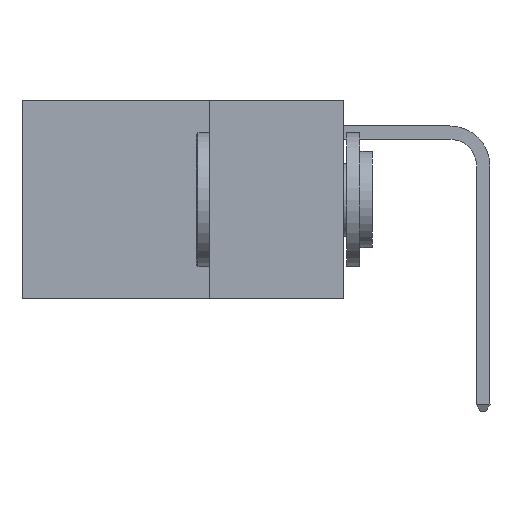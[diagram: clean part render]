
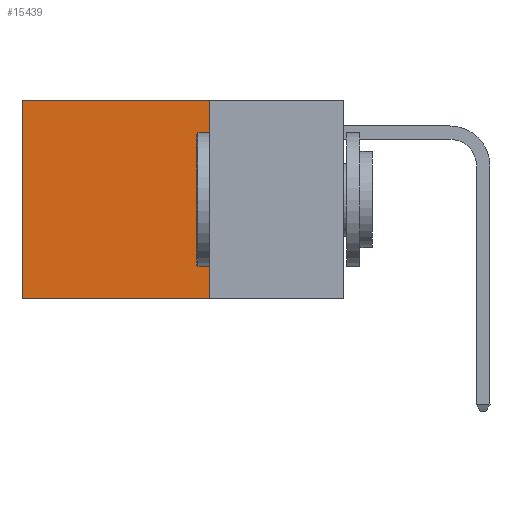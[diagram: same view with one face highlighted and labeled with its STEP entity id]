
A CAD part, left-side view. The second image highlights one B-rep face of the part: STEP entity #15439.
In plain terms, the highlighted planar face has unit normal (-1, 0, 0).
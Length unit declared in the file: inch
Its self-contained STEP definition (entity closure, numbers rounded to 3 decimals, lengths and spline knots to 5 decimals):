
#199 = LINE ( 'NONE', #15323, #12254 ) ;
#250 = CARTESIAN_POINT ( 'NONE',  ( 0.2625, 0.6, 0. ) ) ;
#273 = CARTESIAN_POINT ( 'NONE',  ( 0.2625, 0.25, -0.37 ) ) ;
#838 = DIRECTION ( 'NONE',  ( 0., 0., -1. ) ) ;
#1771 = DIRECTION ( 'NONE',  ( 0., 0., -1. ) ) ;
#2340 = LINE ( 'NONE', #19093, #7757 ) ;
#2983 = PLANE ( 'NONE',  #5856 ) ;
#3521 = ORIENTED_EDGE ( 'NONE', *, *, #11851, .T. ) ;
#4267 = VECTOR ( 'NONE', #9124, 39.37008 ) ;
#4502 = LINE ( 'NONE', #16794, #4267 ) ;
#5856 = AXIS2_PLACEMENT_3D ( 'NONE', #6195, #12149, #1771 ) ;
#5955 = EDGE_CURVE ( 'NONE', #17725, #19535, #2340, .T. ) ;
#6195 = CARTESIAN_POINT ( 'NONE',  ( 0.2625, 0.25, 0. ) ) ;
#6237 = VERTEX_POINT ( 'NONE', #6361 ) ;
#6361 = CARTESIAN_POINT ( 'NONE',  ( 0.2625, 0.6, -0.37 ) ) ;
#7359 = ORIENTED_EDGE ( 'NONE', *, *, #14576, .T. ) ;
#7757 = VECTOR ( 'NONE', #838, 39.37008 ) ;
#7917 = LINE ( 'NONE', #250, #14893 ) ;
#8230 = CARTESIAN_POINT ( 'NONE',  ( 0.2625, 0.25, 0. ) ) ;
#8468 = VERTEX_POINT ( 'NONE', #8598 ) ;
#8598 = CARTESIAN_POINT ( 'NONE',  ( 0.2625, 0.6, 0. ) ) ;
#9124 = DIRECTION ( 'NONE',  ( 0., 1., 0. ) ) ;
#10636 = FACE_OUTER_BOUND ( 'NONE', #10668, .T. ) ;
#10668 = EDGE_LOOP ( 'NONE', ( #3521, #18049, #18006, #7359 ) ) ;
#11851 = EDGE_CURVE ( 'NONE', #8468, #6237, #7917, .T. ) ;
#12149 = DIRECTION ( 'NONE',  ( 1., 0., 0. ) ) ;
#12254 = VECTOR ( 'NONE', #18568, 39.37008 ) ;
#12838 = DIRECTION ( 'NONE',  ( 0., 0., -1. ) ) ;
#14576 = EDGE_CURVE ( 'NONE', #17725, #8468, #199, .T. ) ;
#14893 = VECTOR ( 'NONE', #12838, 39.37008 ) ;
#15323 = CARTESIAN_POINT ( 'NONE',  ( 0.2625, 0.25, 0. ) ) ;
#15439 = ADVANCED_FACE ( 'NONE', ( #10636 ), #2983, .F. ) ;
#15513 = EDGE_CURVE ( 'NONE', #19535, #6237, #4502, .T. ) ;
#16794 = CARTESIAN_POINT ( 'NONE',  ( 0.2625, 0.25, -0.37 ) ) ;
#17725 = VERTEX_POINT ( 'NONE', #8230 ) ;
#18006 = ORIENTED_EDGE ( 'NONE', *, *, #5955, .F. ) ;
#18049 = ORIENTED_EDGE ( 'NONE', *, *, #15513, .F. ) ;
#18568 = DIRECTION ( 'NONE',  ( 0., 1., 0. ) ) ;
#19093 = CARTESIAN_POINT ( 'NONE',  ( 0.2625, 0.25, 0. ) ) ;
#19535 = VERTEX_POINT ( 'NONE', #273 ) ;
